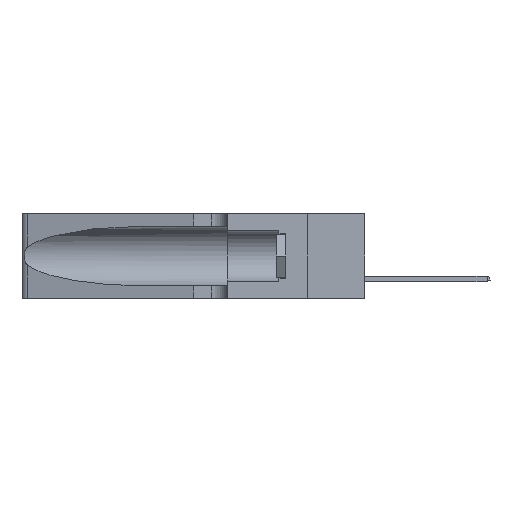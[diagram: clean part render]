
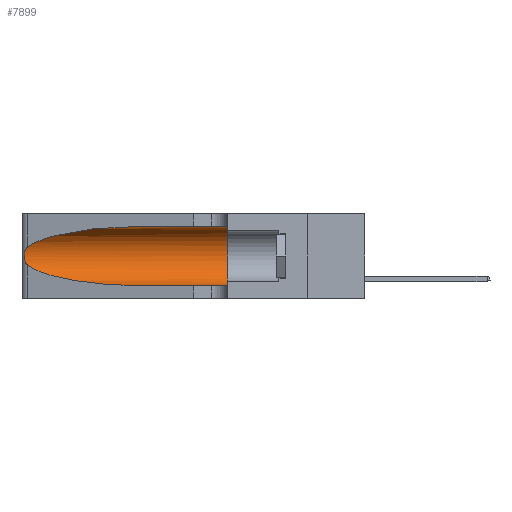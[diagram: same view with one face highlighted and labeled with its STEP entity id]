
A CAD part, left-side view. The second image highlights one B-rep face of the part: STEP entity #7899.
In plain terms, the highlighted cylindrical face has radius 3.308 mm (diameter 6.617 mm), a partial arc.
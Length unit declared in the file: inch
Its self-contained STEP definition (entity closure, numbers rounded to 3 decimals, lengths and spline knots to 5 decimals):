
#443 = CARTESIAN_POINT ( 'NONE',  ( 0.26075, 1.23896, 0.178 ) ) ;
#539 = CARTESIAN_POINT ( 'NONE',  ( 0.25639, 1.23184, 0.21858 ) ) ;
#647 = CARTESIAN_POINT ( 'NONE',  ( 0.25856, 1.23593, 0.16098 ) ) ;
#847 = VERTEX_POINT ( 'NONE', #27782 ) ;
#891 = AXIS2_PLACEMENT_3D ( 'NONE', #26521, #1571, #15176 ) ;
#1077 = CARTESIAN_POINT ( 'NONE',  ( 0.2373, 1.15595, 0.28018 ) ) ;
#1231 = DIRECTION ( 'NONE',  ( 0., -1., 0. ) ) ;
#1571 = DIRECTION ( 'NONE',  ( 0., 1., 0. ) ) ;
#2067 = ORIENTED_EDGE ( 'NONE', *, *, #17066, .T. ) ;
#2105 = ORIENTED_EDGE ( 'NONE', *, *, #6955, .F. ) ;
#2433 = VECTOR ( 'NONE', #13318, 39.37008 ) ;
#2667 = ORIENTED_EDGE ( 'NONE', *, *, #21776, .T. ) ;
#2725 = CARTESIAN_POINT ( 'NONE',  ( 0.25487, 1.22718, 0.14631 ) ) ;
#3454 = CARTESIAN_POINT ( 'NONE',  ( 0.25487, 1.22718, 0.22369 ) ) ;
#4270 = EDGE_CURVE ( 'NONE', #11347, #847, #25567, .T. ) ;
#4743 = VERTEX_POINT ( 'NONE', #22092 ) ;
#5807 = B_SPLINE_CURVE_WITH_KNOTS ( 'NONE', 3,
 ( #6880, #6602, #539, #7340, #16141, #18399, #7061, #443, #25409, #647, #23307, #25601, #20895, #2725 ),
 .UNSPECIFIED., .F., .F.,
 ( 4, 2, 2, 2, 2, 2, 4 ),
 ( 0., 0.00027, 0.00053, 0.00107, 0.0016, 0.00187, 0.00214 ),
 .UNSPECIFIED. ) ;
#5999 = VERTEX_POINT ( 'NONE', #10064 ) ;
#6197 = CIRCLE ( 'NONE', #891, 0.13025 ) ;
#6203 =( BOUNDED_CURVE ( )  B_SPLINE_CURVE ( 3, ( #26772, #10825, #24179, #12831 ),
 .UNSPECIFIED., .F., .T. ) 
 B_SPLINE_CURVE_WITH_KNOTS ( ( 4, 4 ),
 ( 3.44316, 4.71239 ),
 .UNSPECIFIED. ) 
 CURVE ( )  GEOMETRIC_REPRESENTATION_ITEM ( )  RATIONAL_B_SPLINE_CURVE ( ( 1., 0.87, 0.87, 1. ) ) 
 REPRESENTATION_ITEM ( '' )  );
#6602 = CARTESIAN_POINT ( 'NONE',  ( 0.25555, 1.22994, 0.2215 ) ) ;
#6757 = EDGE_LOOP ( 'NONE', ( #27356, #2067, #2667, #26363, #2105, #15231 ) ) ;
#6836 = EDGE_CURVE ( 'NONE', #11347, #4743, #13840, .T. ) ;
#6880 = CARTESIAN_POINT ( 'NONE',  ( 0.25487, 1.22718, 0.22369 ) ) ;
#6955 = EDGE_CURVE ( 'NONE', #847, #12127, #6197, .T. ) ;
#7061 = CARTESIAN_POINT ( 'NONE',  ( 0.26075, 1.23896, 0.19203 ) ) ;
#7321 = VECTOR ( 'NONE', #1231, 39.37008 ) ;
#7340 = CARTESIAN_POINT ( 'NONE',  ( 0.25787, 1.23484, 0.2124 ) ) ;
#7527 = CYLINDRICAL_SURFACE ( 'NONE', #18025, 0.13025 ) ;
#7899 = ADVANCED_FACE ( 'NONE', ( #21061 ), #7527, .F. ) ;
#9573 = DIRECTION ( 'NONE',  ( 0., 0., -1. ) ) ;
#10064 = CARTESIAN_POINT ( 'NONE',  ( 0.25487, 1.22718, 0.14631 ) ) ;
#10252 = CARTESIAN_POINT ( 'NONE',  ( 0.1305, 0.72297, 0.31525 ) ) ;
#10299 = CARTESIAN_POINT ( 'NONE',  ( 0.1305, 1.61858, 0.05475 ) ) ;
#10825 = CARTESIAN_POINT ( 'NONE',  ( 0.2373, 1.15595, 0.08982 ) ) ;
#11347 = VERTEX_POINT ( 'NONE', #13105 ) ;
#11979 = LINE ( 'NONE', #10299, #7321 ) ;
#12127 = VERTEX_POINT ( 'NONE', #16694 ) ;
#12831 = CARTESIAN_POINT ( 'NONE',  ( 0.1305, 0.72297, 0.05475 ) ) ;
#13105 = CARTESIAN_POINT ( 'NONE',  ( 0.1305, 0.72297, 0.31525 ) ) ;
#13318 = DIRECTION ( 'NONE',  ( 0., -1., 0. ) ) ;
#13840 =( BOUNDED_CURVE ( )  B_SPLINE_CURVE ( 3, ( #10252, #14681, #1077, #3454 ),
 .UNSPECIFIED., .F., .F. ) 
 B_SPLINE_CURVE_WITH_KNOTS ( ( 4, 4 ),
 ( 1.5708, 2.84003 ),
 .UNSPECIFIED. ) 
 CURVE ( )  GEOMETRIC_REPRESENTATION_ITEM ( )  RATIONAL_B_SPLINE_CURVE ( ( 1., 0.87, 0.87, 1. ) ) 
 REPRESENTATION_ITEM ( '' )  );
#14114 = DIRECTION ( 'NONE',  ( 0., -1., 0. ) ) ;
#14681 = CARTESIAN_POINT ( 'NONE',  ( 0.18966, 0.96281, 0.31525 ) ) ;
#15176 = DIRECTION ( 'NONE',  ( 0., 0., 1. ) ) ;
#15231 = ORIENTED_EDGE ( 'NONE', *, *, #4270, .F. ) ;
#16063 = CARTESIAN_POINT ( 'NONE',  ( 0.1305, 0.72297, 0.05475 ) ) ;
#16141 = CARTESIAN_POINT ( 'NONE',  ( 0.25854, 1.2359, 0.20912 ) ) ;
#16694 = CARTESIAN_POINT ( 'NONE',  ( 0.1305, 0.35, 0.05475 ) ) ;
#17066 = EDGE_CURVE ( 'NONE', #4743, #5999, #5807, .T. ) ;
#18025 = AXIS2_PLACEMENT_3D ( 'NONE', #18945, #14114, #9573 ) ;
#18399 = CARTESIAN_POINT ( 'NONE',  ( 0.26018, 1.23835, 0.19895 ) ) ;
#18945 = CARTESIAN_POINT ( 'NONE',  ( 0.1305, 1.61858, 0.185 ) ) ;
#20895 = CARTESIAN_POINT ( 'NONE',  ( 0.25555, 1.22993, 0.14849 ) ) ;
#21061 = FACE_OUTER_BOUND ( 'NONE', #6757, .T. ) ;
#21695 = EDGE_CURVE ( 'NONE', #27272, #12127, #11979, .T. ) ;
#21776 = EDGE_CURVE ( 'NONE', #5999, #27272, #6203, .T. ) ;
#22092 = CARTESIAN_POINT ( 'NONE',  ( 0.25487, 1.22718, 0.22369 ) ) ;
#23307 = CARTESIAN_POINT ( 'NONE',  ( 0.25789, 1.23486, 0.15765 ) ) ;
#24179 = CARTESIAN_POINT ( 'NONE',  ( 0.18966, 0.96281, 0.05475 ) ) ;
#25409 = CARTESIAN_POINT ( 'NONE',  ( 0.26017, 1.23833, 0.17102 ) ) ;
#25567 = LINE ( 'NONE', #26839, #2433 ) ;
#25601 = CARTESIAN_POINT ( 'NONE',  ( 0.25639, 1.23186, 0.15144 ) ) ;
#26363 = ORIENTED_EDGE ( 'NONE', *, *, #21695, .T. ) ;
#26521 = CARTESIAN_POINT ( 'NONE',  ( 0.1305, 0.35, 0.185 ) ) ;
#26772 = CARTESIAN_POINT ( 'NONE',  ( 0.25487, 1.22718, 0.14631 ) ) ;
#26839 = CARTESIAN_POINT ( 'NONE',  ( 0.1305, 1.61858, 0.31525 ) ) ;
#27272 = VERTEX_POINT ( 'NONE', #16063 ) ;
#27356 = ORIENTED_EDGE ( 'NONE', *, *, #6836, .T. ) ;
#27782 = CARTESIAN_POINT ( 'NONE',  ( 0.1305, 0.35, 0.31525 ) ) ;
